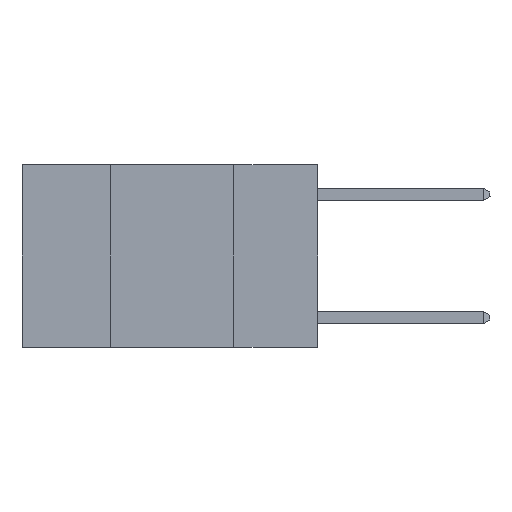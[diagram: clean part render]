
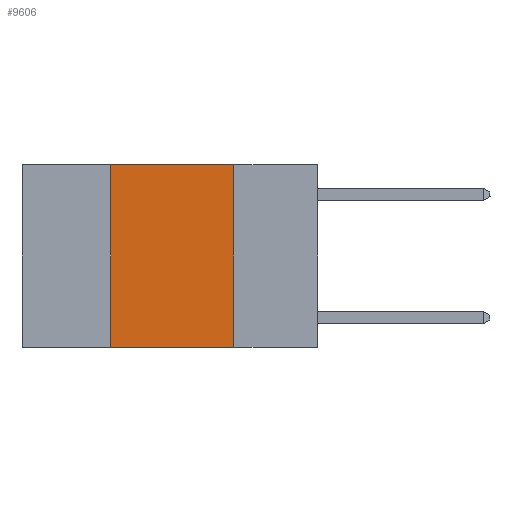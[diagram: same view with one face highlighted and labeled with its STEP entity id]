
A CAD part, left-side view. The second image highlights one B-rep face of the part: STEP entity #9606.
In plain terms, the highlighted planar face has unit normal (-1, 0, 0).
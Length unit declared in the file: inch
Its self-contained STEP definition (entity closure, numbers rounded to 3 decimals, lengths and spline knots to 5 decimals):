
#185 = ORIENTED_EDGE ( 'NONE', *, *, #12678, .T. ) ;
#226 = PLANE ( 'NONE',  #8003 ) ;
#2226 = VECTOR ( 'NONE', #15946, 39.37008 ) ;
#2258 = VERTEX_POINT ( 'NONE', #13229 ) ;
#2775 = DIRECTION ( 'NONE',  ( 0., 0., 1. ) ) ;
#3903 = LINE ( 'NONE', #7372, #2226 ) ;
#3990 = ORIENTED_EDGE ( 'NONE', *, *, #20996, .F. ) ;
#4171 = DIRECTION ( 'NONE',  ( 0., -1., 0. ) ) ;
#4802 = EDGE_CURVE ( 'NONE', #20849, #15508, #11565, .T. ) ;
#5894 = LINE ( 'NONE', #16554, #10930 ) ;
#5969 = DIRECTION ( 'NONE',  ( 0., 0., -1. ) ) ;
#6128 = EDGE_CURVE ( 'NONE', #15508, #20487, #5894, .T. ) ;
#6201 = DIRECTION ( 'NONE',  ( 1., 0., 0. ) ) ;
#7034 = ORIENTED_EDGE ( 'NONE', *, *, #6128, .F. ) ;
#7245 = CARTESIAN_POINT ( 'NONE',  ( 0., 0.6, 0. ) ) ;
#7372 = CARTESIAN_POINT ( 'NONE',  ( 0., 0.6, -0.37 ) ) ;
#8003 = AXIS2_PLACEMENT_3D ( 'NONE', #7245, #6201, #5969 ) ;
#8991 = FACE_OUTER_BOUND ( 'NONE', #13817, .T. ) ;
#9606 = ADVANCED_FACE ( 'NONE', ( #8991 ), #226, .F. ) ;
#9933 = CARTESIAN_POINT ( 'NONE',  ( 0., 0.42, 0. ) ) ;
#10930 = VECTOR ( 'NONE', #4171, 39.37008 ) ;
#11565 = LINE ( 'NONE', #9933, #19757 ) ;
#12678 = EDGE_CURVE ( 'NONE', #20849, #2258, #3903, .T. ) ;
#13229 = CARTESIAN_POINT ( 'NONE',  ( 0., 0.17, -0.37 ) ) ;
#13817 = EDGE_LOOP ( 'NONE', ( #3990, #7034, #16476, #185 ) ) ;
#14535 = DIRECTION ( 'NONE',  ( 0., 0., -1. ) ) ;
#15508 = VERTEX_POINT ( 'NONE', #22218 ) ;
#15946 = DIRECTION ( 'NONE',  ( 0., -1., 0. ) ) ;
#16090 = CARTESIAN_POINT ( 'NONE',  ( 0., 0.17, 0. ) ) ;
#16476 = ORIENTED_EDGE ( 'NONE', *, *, #4802, .F. ) ;
#16554 = CARTESIAN_POINT ( 'NONE',  ( 0., 0.6, 0. ) ) ;
#17533 = VECTOR ( 'NONE', #14535, 39.37008 ) ;
#19516 = LINE ( 'NONE', #21375, #17533 ) ;
#19757 = VECTOR ( 'NONE', #2775, 39.37008 ) ;
#20487 = VERTEX_POINT ( 'NONE', #16090 ) ;
#20685 = CARTESIAN_POINT ( 'NONE',  ( 0., 0.42, -0.37 ) ) ;
#20849 = VERTEX_POINT ( 'NONE', #20685 ) ;
#20996 = EDGE_CURVE ( 'NONE', #20487, #2258, #19516, .T. ) ;
#21375 = CARTESIAN_POINT ( 'NONE',  ( 0., 0.17, 0. ) ) ;
#22218 = CARTESIAN_POINT ( 'NONE',  ( 0., 0.42, 0. ) ) ;
